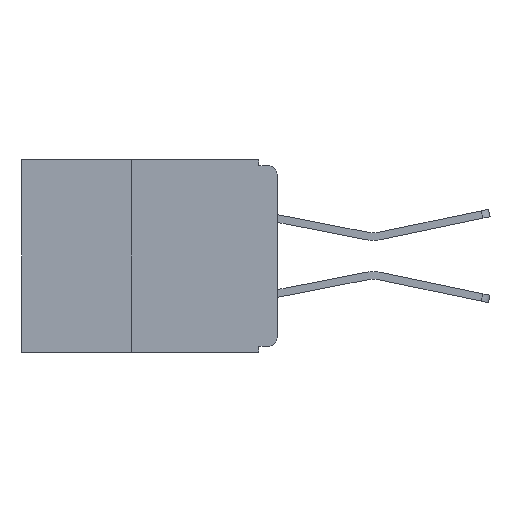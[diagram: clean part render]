
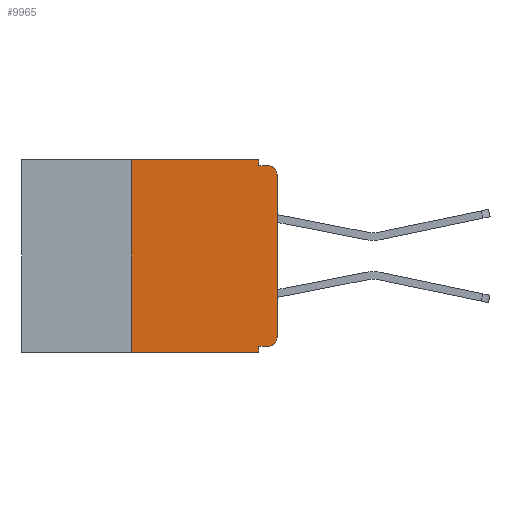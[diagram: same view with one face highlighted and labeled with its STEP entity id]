
A CAD part, left-side view. The second image highlights one B-rep face of the part: STEP entity #9965.
In plain terms, the highlighted planar face has unit normal (-1, 0, 0).
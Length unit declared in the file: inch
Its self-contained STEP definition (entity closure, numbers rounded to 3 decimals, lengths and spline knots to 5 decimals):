
#283 = VERTEX_POINT ( 'NONE', #22951 ) ;
#615 = LINE ( 'NONE', #12561, #11023 ) ;
#683 = DIRECTION ( 'NONE',  ( 1., 0., 0. ) ) ;
#951 = EDGE_CURVE ( 'NONE', #6304, #9585, #615, .T. ) ;
#1410 = ORIENTED_EDGE ( 'NONE', *, *, #22751, .T. ) ;
#1633 = DIRECTION ( 'NONE',  ( 0., 0., 1. ) ) ;
#1868 = CARTESIAN_POINT ( 'NONE',  ( 0., 0.25, -0.33 ) ) ;
#1903 = CARTESIAN_POINT ( 'NONE',  ( 0., 0.031, 0. ) ) ;
#2288 = LINE ( 'NONE', #5391, #7252 ) ;
#2325 = VERTEX_POINT ( 'NONE', #15751 ) ;
#2444 = EDGE_CURVE ( 'NONE', #2325, #283, #19767, .T. ) ;
#3313 = EDGE_CURVE ( 'NONE', #3782, #2325, #14696, .T. ) ;
#3782 = VERTEX_POINT ( 'NONE', #24708 ) ;
#4174 = EDGE_CURVE ( 'NONE', #20705, #11347, #11155, .T. ) ;
#4329 = VECTOR ( 'NONE', #7087, 39.37008 ) ;
#4488 = CARTESIAN_POINT ( 'NONE',  ( 0., 0.015, -0.01 ) ) ;
#5153 = EDGE_CURVE ( 'NONE', #9585, #9349, #15222, .T. ) ;
#5391 = CARTESIAN_POINT ( 'NONE',  ( 0., 0.437, -0.33 ) ) ;
#5760 = ORIENTED_EDGE ( 'NONE', *, *, #3313, .F. ) ;
#5870 = FACE_OUTER_BOUND ( 'NONE', #13107, .T. ) ;
#6304 = VERTEX_POINT ( 'NONE', #1903 ) ;
#6599 = CIRCLE ( 'NONE', #7070, 0.015 ) ;
#7032 = CARTESIAN_POINT ( 'NONE',  ( 0., 0., -0.01 ) ) ;
#7044 = ORIENTED_EDGE ( 'NONE', *, *, #5153, .F. ) ;
#7070 = AXIS2_PLACEMENT_3D ( 'NONE', #23386, #11414, #25377 ) ;
#7087 = DIRECTION ( 'NONE',  ( 0., -1., 0. ) ) ;
#7222 = CARTESIAN_POINT ( 'NONE',  ( 0., 0.015, -0.025 ) ) ;
#7252 = VECTOR ( 'NONE', #19589, 39.37008 ) ;
#7736 = ORIENTED_EDGE ( 'NONE', *, *, #23966, .T. ) ;
#8174 = VECTOR ( 'NONE', #20603, 39.37008 ) ;
#8223 = EDGE_CURVE ( 'NONE', #20567, #21519, #16346, .T. ) ;
#8573 = CARTESIAN_POINT ( 'NONE',  ( 0., 0.437, 0. ) ) ;
#9306 = DIRECTION ( 'NONE',  ( 0., 0., -1. ) ) ;
#9333 = ORIENTED_EDGE ( 'NONE', *, *, #951, .F. ) ;
#9349 = VERTEX_POINT ( 'NONE', #4488 ) ;
#9585 = VERTEX_POINT ( 'NONE', #25457 ) ;
#9618 = AXIS2_PLACEMENT_3D ( 'NONE', #25017, #683, #15114 ) ;
#9960 = ORIENTED_EDGE ( 'NONE', *, *, #2444, .F. ) ;
#9965 = ADVANCED_FACE ( 'NONE', ( #5870 ), #13078, .F. ) ;
#10963 = VECTOR ( 'NONE', #1633, 39.37008 ) ;
#11023 = VECTOR ( 'NONE', #26193, 39.37008 ) ;
#11155 = LINE ( 'NONE', #19610, #20602 ) ;
#11347 = VERTEX_POINT ( 'NONE', #13166 ) ;
#11414 = DIRECTION ( 'NONE',  ( -1., 0., 0. ) ) ;
#12561 = CARTESIAN_POINT ( 'NONE',  ( 0., 0.031, 0. ) ) ;
#13078 = PLANE ( 'NONE',  #9618 ) ;
#13107 = EDGE_LOOP ( 'NONE', ( #19980, #1410, #7044, #9333, #21237, #24949, #16894, #9960, #5760, #7736 ) ) ;
#13166 = CARTESIAN_POINT ( 'NONE',  ( 0., 0., -0.025 ) ) ;
#13591 = DIRECTION ( 'NONE',  ( 0., 0., -1. ) ) ;
#13687 = CARTESIAN_POINT ( 'NONE',  ( 0., 0.031, -0.33 ) ) ;
#13948 = CARTESIAN_POINT ( 'NONE',  ( 0., 0., -0.32 ) ) ;
#13954 = DIRECTION ( 'NONE',  ( 0., 1., 0. ) ) ;
#14430 = VECTOR ( 'NONE', #13591, 39.37008 ) ;
#14696 = LINE ( 'NONE', #13948, #24651 ) ;
#15114 = DIRECTION ( 'NONE',  ( 0., 0., -1. ) ) ;
#15177 = EDGE_CURVE ( 'NONE', #20567, #283, #2288, .T. ) ;
#15222 = LINE ( 'NONE', #7032, #4329 ) ;
#15751 = CARTESIAN_POINT ( 'NONE',  ( 0., 0.031, -0.32 ) ) ;
#16346 = LINE ( 'NONE', #1868, #10963 ) ;
#16894 = ORIENTED_EDGE ( 'NONE', *, *, #15177, .T. ) ;
#18530 = EDGE_CURVE ( 'NONE', #21519, #6304, #18895, .T. ) ;
#18895 = LINE ( 'NONE', #8573, #8174 ) ;
#19070 = AXIS2_PLACEMENT_3D ( 'NONE', #7222, #21297, #9306 ) ;
#19589 = DIRECTION ( 'NONE',  ( 0., -1., 0. ) ) ;
#19610 = CARTESIAN_POINT ( 'NONE',  ( 0., 0., 0. ) ) ;
#19686 = CARTESIAN_POINT ( 'NONE',  ( 0., 0.25, 0. ) ) ;
#19728 = DIRECTION ( 'NONE',  ( 0., 0., 1. ) ) ;
#19767 = LINE ( 'NONE', #13687, #14430 ) ;
#19980 = ORIENTED_EDGE ( 'NONE', *, *, #4174, .T. ) ;
#20252 = CARTESIAN_POINT ( 'NONE',  ( 0., 0.25, -0.33 ) ) ;
#20567 = VERTEX_POINT ( 'NONE', #20252 ) ;
#20602 = VECTOR ( 'NONE', #19728, 39.37008 ) ;
#20603 = DIRECTION ( 'NONE',  ( 0., -1., 0. ) ) ;
#20705 = VERTEX_POINT ( 'NONE', #22647 ) ;
#20889 = CIRCLE ( 'NONE', #19070, 0.015 ) ;
#21237 = ORIENTED_EDGE ( 'NONE', *, *, #18530, .F. ) ;
#21297 = DIRECTION ( 'NONE',  ( -1., 0., 0. ) ) ;
#21519 = VERTEX_POINT ( 'NONE', #19686 ) ;
#22647 = CARTESIAN_POINT ( 'NONE',  ( 0., 0., -0.305 ) ) ;
#22751 = EDGE_CURVE ( 'NONE', #11347, #9349, #20889, .T. ) ;
#22951 = CARTESIAN_POINT ( 'NONE',  ( 0., 0.031, -0.33 ) ) ;
#23386 = CARTESIAN_POINT ( 'NONE',  ( 0., 0.015, -0.305 ) ) ;
#23966 = EDGE_CURVE ( 'NONE', #3782, #20705, #6599, .T. ) ;
#24651 = VECTOR ( 'NONE', #13954, 39.37008 ) ;
#24708 = CARTESIAN_POINT ( 'NONE',  ( 0., 0.015, -0.32 ) ) ;
#24949 = ORIENTED_EDGE ( 'NONE', *, *, #8223, .F. ) ;
#25017 = CARTESIAN_POINT ( 'NONE',  ( 0., 0.437, 0. ) ) ;
#25377 = DIRECTION ( 'NONE',  ( 0., 0., -1. ) ) ;
#25457 = CARTESIAN_POINT ( 'NONE',  ( 0., 0.031, -0.01 ) ) ;
#26193 = DIRECTION ( 'NONE',  ( 0., 0., -1. ) ) ;
